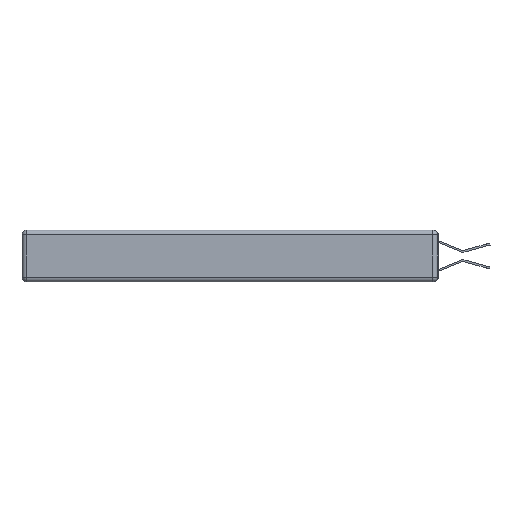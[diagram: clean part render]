
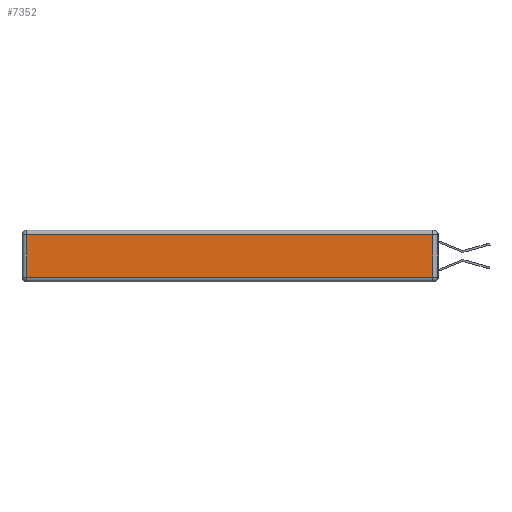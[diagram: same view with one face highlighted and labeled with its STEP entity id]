
A CAD part, left-side view. The second image highlights one B-rep face of the part: STEP entity #7352.
In plain terms, the highlighted planar face has unit normal (-1, 0, 0).
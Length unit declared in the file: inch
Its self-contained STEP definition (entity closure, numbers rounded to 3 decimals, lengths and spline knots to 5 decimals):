
#831 = VECTOR ( 'NONE', #3359, 39.37008 ) ;
#912 = ORIENTED_EDGE ( 'NONE', *, *, #13434, .T. ) ;
#931 = EDGE_CURVE ( 'NONE', #1211, #11239, #11241, .T. ) ;
#1175 = FACE_OUTER_BOUND ( 'NONE', #11243, .T. ) ;
#1211 = VERTEX_POINT ( 'NONE', #7749 ) ;
#1954 = AXIS2_PLACEMENT_3D ( 'NONE', #13796, #13585, #6058 ) ;
#2357 = CARTESIAN_POINT ( 'NONE',  ( 0., 2.75, -0.03 ) ) ;
#2660 = LINE ( 'NONE', #9080, #7308 ) ;
#3359 = DIRECTION ( 'NONE',  ( 0., 1., 0. ) ) ;
#3556 = CARTESIAN_POINT ( 'NONE',  ( 0., 2.72, -0.343 ) ) ;
#3849 = LINE ( 'NONE', #6854, #4743 ) ;
#4743 = VECTOR ( 'NONE', #9187, 39.37008 ) ;
#5530 = CARTESIAN_POINT ( 'NONE',  ( 0., 2.72, -0.313 ) ) ;
#5633 = CARTESIAN_POINT ( 'NONE',  ( 0., 0.03, -0.313 ) ) ;
#5872 = VERTEX_POINT ( 'NONE', #5633 ) ;
#6058 = DIRECTION ( 'NONE',  ( 0., 0., 1. ) ) ;
#6785 = DIRECTION ( 'NONE',  ( 0., 0., -1. ) ) ;
#6854 = CARTESIAN_POINT ( 'NONE',  ( 0., 0., -0.313 ) ) ;
#7308 = VECTOR ( 'NONE', #8220, 39.37008 ) ;
#7352 = ADVANCED_FACE ( 'NONE', ( #1175 ), #11000, .T. ) ;
#7749 = CARTESIAN_POINT ( 'NONE',  ( 0., 2.72, -0.03 ) ) ;
#8155 = CARTESIAN_POINT ( 'NONE',  ( 0., 0.03, -0.03 ) ) ;
#8220 = DIRECTION ( 'NONE',  ( 0., 0., 1. ) ) ;
#8388 = EDGE_CURVE ( 'NONE', #5872, #10973, #2660, .T. ) ;
#8922 = LINE ( 'NONE', #2357, #831 ) ;
#9080 = CARTESIAN_POINT ( 'NONE',  ( 0., 0.03, -0.343 ) ) ;
#9187 = DIRECTION ( 'NONE',  ( 0., -1., 0. ) ) ;
#9263 = ORIENTED_EDGE ( 'NONE', *, *, #8388, .T. ) ;
#9970 = EDGE_CURVE ( 'NONE', #10973, #1211, #8922, .T. ) ;
#10973 = VERTEX_POINT ( 'NONE', #8155 ) ;
#11000 = PLANE ( 'NONE',  #1954 ) ;
#11239 = VERTEX_POINT ( 'NONE', #5530 ) ;
#11241 = LINE ( 'NONE', #3556, #12003 ) ;
#11243 = EDGE_LOOP ( 'NONE', ( #912, #9263, #13485, #12693 ) ) ;
#12003 = VECTOR ( 'NONE', #6785, 39.37008 ) ;
#12693 = ORIENTED_EDGE ( 'NONE', *, *, #931, .T. ) ;
#13434 = EDGE_CURVE ( 'NONE', #11239, #5872, #3849, .T. ) ;
#13485 = ORIENTED_EDGE ( 'NONE', *, *, #9970, .T. ) ;
#13585 = DIRECTION ( 'NONE',  ( -1., 0., 0. ) ) ;
#13796 = CARTESIAN_POINT ( 'NONE',  ( 0., 0., -0.343 ) ) ;
